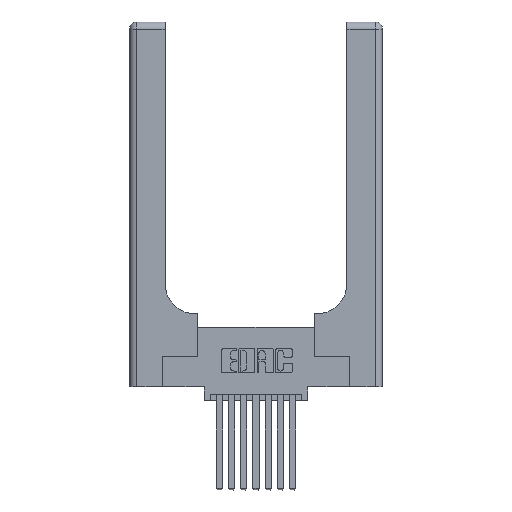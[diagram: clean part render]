
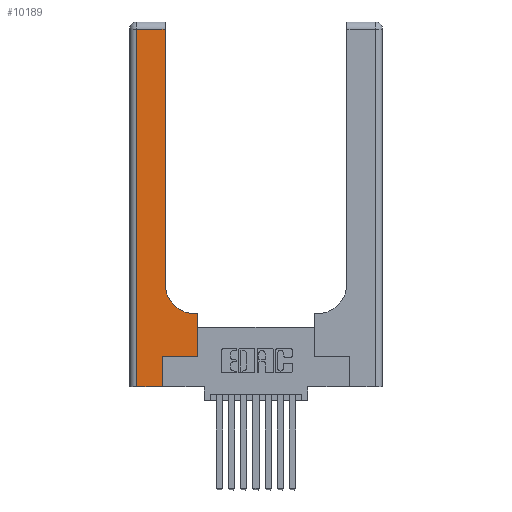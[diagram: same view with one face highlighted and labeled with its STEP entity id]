
A CAD part, top view. The second image highlights one B-rep face of the part: STEP entity #10189.
In plain terms, the highlighted planar face has unit normal (0, 0, 1).
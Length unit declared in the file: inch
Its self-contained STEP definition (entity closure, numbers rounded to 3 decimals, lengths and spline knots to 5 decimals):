
#509 = VERTEX_POINT ( 'NONE', #3077 ) ;
#576 = VERTEX_POINT ( 'NONE', #10631 ) ;
#607 = CARTESIAN_POINT ( 'NONE',  ( 0.06, 3., 0.37 ) ) ;
#623 = ORIENTED_EDGE ( 'NONE', *, *, #1325, .T. ) ;
#762 = DIRECTION ( 'NONE',  ( 1., 0., 0. ) ) ;
#1325 = EDGE_CURVE ( 'NONE', #8862, #7503, #3499, .T. ) ;
#1546 = CARTESIAN_POINT ( 'NONE',  ( 0.2915, 3., 0.37 ) ) ;
#1594 = ORIENTED_EDGE ( 'NONE', *, *, #2685, .T. ) ;
#1640 = EDGE_CURVE ( 'NONE', #3384, #8862, #6878, .T. ) ;
#1759 = AXIS2_PLACEMENT_3D ( 'NONE', #12723, #15045, #8203 ) ;
#1817 = VECTOR ( 'NONE', #7928, 39.37008 ) ;
#1844 = CARTESIAN_POINT ( 'NONE',  ( 0.2915, 2.94, 0.37 ) ) ;
#1980 = ORIENTED_EDGE ( 'NONE', *, *, #12104, .T. ) ;
#2038 = CARTESIAN_POINT ( 'NONE',  ( 0.269, 0.25, 0.37 ) ) ;
#2311 = AXIS2_PLACEMENT_3D ( 'NONE', #10287, #9466, #8898 ) ;
#2443 = LINE ( 'NONE', #7026, #2828 ) ;
#2538 = CARTESIAN_POINT ( 'NONE',  ( 0.269, 0., 0.37 ) ) ;
#2685 = EDGE_CURVE ( 'NONE', #7518, #3384, #3660, .T. ) ;
#2828 = VECTOR ( 'NONE', #7012, 39.37008 ) ;
#3046 = ORIENTED_EDGE ( 'NONE', *, *, #3197, .T. ) ;
#3077 = CARTESIAN_POINT ( 'NONE',  ( 0.06, 2.94, 0.37 ) ) ;
#3197 = EDGE_CURVE ( 'NONE', #7503, #509, #2443, .T. ) ;
#3384 = VERTEX_POINT ( 'NONE', #5411 ) ;
#3499 = LINE ( 'NONE', #1546, #9454 ) ;
#3505 = EDGE_LOOP ( 'NONE', ( #623, #3046, #7089, #1980, #8093, #7131, #3971, #1594, #6735 ) ) ;
#3605 = DIRECTION ( 'NONE',  ( 0., 1., 0. ) ) ;
#3660 = LINE ( 'NONE', #11213, #12267 ) ;
#3841 = VECTOR ( 'NONE', #762, 39.37008 ) ;
#3971 = ORIENTED_EDGE ( 'NONE', *, *, #7736, .T. ) ;
#4029 = CARTESIAN_POINT ( 'NONE',  ( 0., 0., 0.37 ) ) ;
#5218 = DIRECTION ( 'NONE',  ( 1., 0., 0. ) ) ;
#5411 = CARTESIAN_POINT ( 'NONE',  ( 0.5415, 0.6, 0.37 ) ) ;
#6735 = ORIENTED_EDGE ( 'NONE', *, *, #1640, .T. ) ;
#6800 = VECTOR ( 'NONE', #3605, 39.37008 ) ;
#6878 = CIRCLE ( 'NONE', #2311, 0.25 ) ;
#6941 = FACE_OUTER_BOUND ( 'NONE', #3505, .T. ) ;
#6973 = EDGE_CURVE ( 'NONE', #8329, #576, #13153, .T. ) ;
#7012 = DIRECTION ( 'NONE',  ( -1., 0., 0. ) ) ;
#7026 = CARTESIAN_POINT ( 'NONE',  ( 0., 2.94, 0.37 ) ) ;
#7089 = ORIENTED_EDGE ( 'NONE', *, *, #8136, .T. ) ;
#7131 = ORIENTED_EDGE ( 'NONE', *, *, #6973, .T. ) ;
#7165 = CARTESIAN_POINT ( 'NONE',  ( 0.5585, 0.25, 0.37 ) ) ;
#7174 = LINE ( 'NONE', #7165, #6800 ) ;
#7237 = CARTESIAN_POINT ( 'NONE',  ( 0.2915, 0.85, 0.37 ) ) ;
#7503 = VERTEX_POINT ( 'NONE', #1844 ) ;
#7518 = VERTEX_POINT ( 'NONE', #12527 ) ;
#7657 = DIRECTION ( 'NONE',  ( 0., 1., 0. ) ) ;
#7736 = EDGE_CURVE ( 'NONE', #576, #7518, #7174, .T. ) ;
#7895 = VERTEX_POINT ( 'NONE', #12159 ) ;
#7928 = DIRECTION ( 'NONE',  ( 0., -1., 0. ) ) ;
#8093 = ORIENTED_EDGE ( 'NONE', *, *, #8314, .T. ) ;
#8136 = EDGE_CURVE ( 'NONE', #509, #14322, #13992, .T. ) ;
#8203 = DIRECTION ( 'NONE',  ( -1., 0., 0. ) ) ;
#8314 = EDGE_CURVE ( 'NONE', #7895, #8329, #8811, .T. ) ;
#8329 = VERTEX_POINT ( 'NONE', #14301 ) ;
#8811 = LINE ( 'NONE', #2538, #11870 ) ;
#8862 = VERTEX_POINT ( 'NONE', #7237 ) ;
#8898 = DIRECTION ( 'NONE',  ( 1., 0., 0. ) ) ;
#9454 = VECTOR ( 'NONE', #7657, 39.37008 ) ;
#9466 = DIRECTION ( 'NONE',  ( 0., 0., -1. ) ) ;
#9563 = LINE ( 'NONE', #4029, #15257 ) ;
#9709 = DIRECTION ( 'NONE',  ( 0., 1., 0. ) ) ;
#10189 = ADVANCED_FACE ( 'NONE', ( #6941 ), #11633, .F. ) ;
#10287 = CARTESIAN_POINT ( 'NONE',  ( 0.5415, 0.85, 0.37 ) ) ;
#10631 = CARTESIAN_POINT ( 'NONE',  ( 0.5585, 0.25, 0.37 ) ) ;
#10997 = CARTESIAN_POINT ( 'NONE',  ( 0.06, 0., 0.37 ) ) ;
#11169 = DIRECTION ( 'NONE',  ( -1., 0., 0. ) ) ;
#11213 = CARTESIAN_POINT ( 'NONE',  ( 0.2915, 0.6, 0.37 ) ) ;
#11633 = PLANE ( 'NONE',  #1759 ) ;
#11870 = VECTOR ( 'NONE', #9709, 39.37008 ) ;
#12104 = EDGE_CURVE ( 'NONE', #14322, #7895, #9563, .T. ) ;
#12159 = CARTESIAN_POINT ( 'NONE',  ( 0.269, 0., 0.37 ) ) ;
#12267 = VECTOR ( 'NONE', #11169, 39.37008 ) ;
#12527 = CARTESIAN_POINT ( 'NONE',  ( 0.5585, 0.6, 0.37 ) ) ;
#12723 = CARTESIAN_POINT ( 'NONE',  ( 0., 3., 0.37 ) ) ;
#13153 = LINE ( 'NONE', #2038, #3841 ) ;
#13992 = LINE ( 'NONE', #607, #1817 ) ;
#14301 = CARTESIAN_POINT ( 'NONE',  ( 0.269, 0.25, 0.37 ) ) ;
#14322 = VERTEX_POINT ( 'NONE', #10997 ) ;
#15045 = DIRECTION ( 'NONE',  ( 0., 0., -1. ) ) ;
#15257 = VECTOR ( 'NONE', #5218, 39.37008 ) ;
